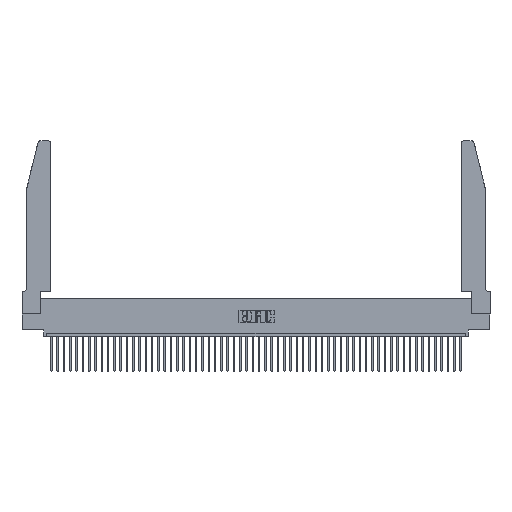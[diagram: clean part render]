
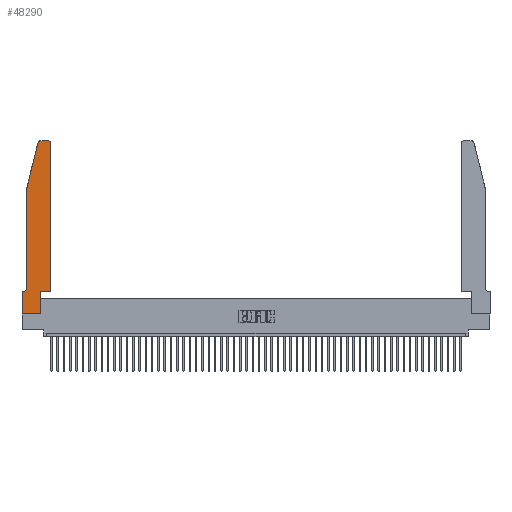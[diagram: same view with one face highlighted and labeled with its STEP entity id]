
A CAD part, top view. The second image highlights one B-rep face of the part: STEP entity #48290.
In plain terms, the highlighted planar face has unit normal (0, 0, 1).
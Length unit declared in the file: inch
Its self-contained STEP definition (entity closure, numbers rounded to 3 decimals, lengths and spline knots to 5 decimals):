
#270 = VECTOR ( 'NONE', #30707, 39.37008 ) ;
#1154 = DIRECTION ( 'NONE',  ( -1., 0., 0. ) ) ;
#1401 = LINE ( 'NONE', #25090, #33498 ) ;
#1733 = CARTESIAN_POINT ( 'NONE',  ( 0.2865, 0.35, 0.37 ) ) ;
#1856 = VERTEX_POINT ( 'NONE', #25695 ) ;
#2236 = DIRECTION ( 'NONE',  ( 1., 0., 0. ) ) ;
#2900 = CARTESIAN_POINT ( 'NONE',  ( 0.0755, 2., 0.37 ) ) ;
#3013 = ORIENTED_EDGE ( 'NONE', *, *, #14143, .T. ) ;
#3440 = DIRECTION ( 'NONE',  ( 0., -1., 0. ) ) ;
#4960 = AXIS2_PLACEMENT_3D ( 'NONE', #7551, #12143, #24899 ) ;
#5431 = EDGE_CURVE ( 'NONE', #17970, #30883, #45743, .T. ) ;
#6636 = DIRECTION ( 'NONE',  ( 0., 0., 1. ) ) ;
#7530 = VERTEX_POINT ( 'NONE', #18806 ) ;
#7551 = CARTESIAN_POINT ( 'NONE',  ( 0.284, 2.72, 0.37 ) ) ;
#8473 = CARTESIAN_POINT ( 'NONE',  ( 0.2605, 2.75, 0.37 ) ) ;
#9824 = ORIENTED_EDGE ( 'NONE', *, *, #10582, .T. ) ;
#10582 = EDGE_CURVE ( 'NONE', #50587, #1856, #40303, .T. ) ;
#10866 = ORIENTED_EDGE ( 'NONE', *, *, #5431, .T. ) ;
#11333 = CARTESIAN_POINT ( 'NONE',  ( 0.0055, 0.42, 0.37 ) ) ;
#12091 = CARTESIAN_POINT ( 'NONE',  ( 0.2865, 0.35, 0.37 ) ) ;
#12143 = DIRECTION ( 'NONE',  ( 0., 0., 1. ) ) ;
#13010 = CARTESIAN_POINT ( 'NONE',  ( 0., 0.35, 0.37 ) ) ;
#13151 = EDGE_CURVE ( 'NONE', #7530, #50587, #1401, .T. ) ;
#13411 = VECTOR ( 'NONE', #21509, 39.37008 ) ;
#13503 = CARTESIAN_POINT ( 'NONE',  ( 0.25487, 2.72718, 0.37 ) ) ;
#13522 = DIRECTION ( 'NONE',  ( 1., 0., 0. ) ) ;
#14143 = EDGE_CURVE ( 'NONE', #32393, #18899, #32865, .T. ) ;
#14717 = DIRECTION ( 'NONE',  ( 0., 0., -1. ) ) ;
#15496 = ORIENTED_EDGE ( 'NONE', *, *, #30659, .T. ) ;
#16083 = CARTESIAN_POINT ( 'NONE',  ( 0.4505, 2.72, 0.37 ) ) ;
#16357 = CARTESIAN_POINT ( 'NONE',  ( 0.0755, 0.42, 0.37 ) ) ;
#16364 = EDGE_CURVE ( 'NONE', #30883, #48592, #29950, .T. ) ;
#16463 = EDGE_CURVE ( 'NONE', #18875, #7530, #46113, .T. ) ;
#16797 = CARTESIAN_POINT ( 'NONE',  ( 0.4205, 2.75, 0.37 ) ) ;
#17970 = VERTEX_POINT ( 'NONE', #22312 ) ;
#18290 = LINE ( 'NONE', #36904, #47576 ) ;
#18806 = CARTESIAN_POINT ( 'NONE',  ( 0.0055, 0.35, 0.37 ) ) ;
#18875 = VERTEX_POINT ( 'NONE', #16357 ) ;
#18899 = VERTEX_POINT ( 'NONE', #48061 ) ;
#19229 = VERTEX_POINT ( 'NONE', #16797 ) ;
#19239 = ORIENTED_EDGE ( 'NONE', *, *, #16463, .T. ) ;
#19717 = CARTESIAN_POINT ( 'NONE',  ( 0.4505, 0.35, 0.37 ) ) ;
#19739 = EDGE_CURVE ( 'NONE', #48592, #18875, #33298, .T. ) ;
#20328 = LINE ( 'NONE', #8473, #27850 ) ;
#20359 = DIRECTION ( 'NONE',  ( 0., -1., 0. ) ) ;
#20773 = EDGE_CURVE ( 'NONE', #1856, #48542, #18290, .T. ) ;
#20975 = CARTESIAN_POINT ( 'NONE',  ( 0., 0.35, 0.37 ) ) ;
#21509 = DIRECTION ( 'NONE',  ( 0., 1., 0. ) ) ;
#21922 = DIRECTION ( 'NONE',  ( 1., 0., 0. ) ) ;
#22312 = CARTESIAN_POINT ( 'NONE',  ( 0.284, 2.75, 0.37 ) ) ;
#22869 = CARTESIAN_POINT ( 'NONE',  ( 0.2865, 0., 0.37 ) ) ;
#23651 = DIRECTION ( 'NONE',  ( -1., 0., 0. ) ) ;
#24859 = ORIENTED_EDGE ( 'NONE', *, *, #16364, .T. ) ;
#24899 = DIRECTION ( 'NONE',  ( 1., 0., 0. ) ) ;
#25090 = CARTESIAN_POINT ( 'NONE',  ( 0.0755, 0.35, 0.37 ) ) ;
#25695 = CARTESIAN_POINT ( 'NONE',  ( 0., 0., 0.37 ) ) ;
#26265 = ORIENTED_EDGE ( 'NONE', *, *, #19739, .T. ) ;
#26430 = AXIS2_PLACEMENT_3D ( 'NONE', #13010, #44469, #33238 ) ;
#27118 = LINE ( 'NONE', #1733, #13411 ) ;
#27508 = VECTOR ( 'NONE', #47598, 39.37008 ) ;
#27850 = VECTOR ( 'NONE', #23651, 39.37008 ) ;
#29950 = LINE ( 'NONE', #2900, #270 ) ;
#30659 = EDGE_CURVE ( 'NONE', #18899, #50947, #45557, .T. ) ;
#30707 = DIRECTION ( 'NONE',  ( -0.239, -0.971, 0. ) ) ;
#30883 = VERTEX_POINT ( 'NONE', #13503 ) ;
#31406 = CARTESIAN_POINT ( 'NONE',  ( 0., 0., 0.37 ) ) ;
#32059 = EDGE_CURVE ( 'NONE', #50947, #19229, #46003, .T. ) ;
#32393 = VERTEX_POINT ( 'NONE', #12091 ) ;
#32865 = LINE ( 'NONE', #33632, #38510 ) ;
#33238 = DIRECTION ( 'NONE',  ( 1., 0., 0. ) ) ;
#33298 = LINE ( 'NONE', #43809, #48322 ) ;
#33498 = VECTOR ( 'NONE', #1154, 39.37008 ) ;
#33632 = CARTESIAN_POINT ( 'NONE',  ( 0.4505, 0.35, 0.37 ) ) ;
#33958 = ORIENTED_EDGE ( 'NONE', *, *, #47804, .T. ) ;
#35311 = ORIENTED_EDGE ( 'NONE', *, *, #32059, .T. ) ;
#36904 = CARTESIAN_POINT ( 'NONE',  ( 0., 0., 0.37 ) ) ;
#37215 = ORIENTED_EDGE ( 'NONE', *, *, #13151, .T. ) ;
#38506 = CARTESIAN_POINT ( 'NONE',  ( 0.0755, 2., 0.37 ) ) ;
#38510 = VECTOR ( 'NONE', #2236, 39.37008 ) ;
#38785 = ORIENTED_EDGE ( 'NONE', *, *, #20773, .T. ) ;
#39945 = ORIENTED_EDGE ( 'NONE', *, *, #46332, .T. ) ;
#40303 = LINE ( 'NONE', #31406, #47049 ) ;
#43061 = DIRECTION ( 'NONE',  ( -1., 0., 0. ) ) ;
#43184 = FACE_OUTER_BOUND ( 'NONE', #43861, .T. ) ;
#43809 = CARTESIAN_POINT ( 'NONE',  ( 0.0755, 2., 0.37 ) ) ;
#43861 = EDGE_LOOP ( 'NONE', ( #39945, #10866, #24859, #26265, #19239, #37215, #9824, #38785, #33958, #3013, #15496, #35311 ) ) ;
#44150 = AXIS2_PLACEMENT_3D ( 'NONE', #11333, #14717, #43061 ) ;
#44469 = DIRECTION ( 'NONE',  ( 0., 0., 1. ) ) ;
#44638 = AXIS2_PLACEMENT_3D ( 'NONE', #50156, #6636, #21922 ) ;
#45557 = LINE ( 'NONE', #19717, #27508 ) ;
#45743 = CIRCLE ( 'NONE', #4960, 0.03 ) ;
#46003 = CIRCLE ( 'NONE', #44638, 0.03 ) ;
#46113 = CIRCLE ( 'NONE', #44150, 0.07 ) ;
#46332 = EDGE_CURVE ( 'NONE', #19229, #17970, #20328, .T. ) ;
#47049 = VECTOR ( 'NONE', #3440, 39.37008 ) ;
#47576 = VECTOR ( 'NONE', #13522, 39.37008 ) ;
#47598 = DIRECTION ( 'NONE',  ( 0., 1., 0. ) ) ;
#47804 = EDGE_CURVE ( 'NONE', #48542, #32393, #27118, .T. ) ;
#48061 = CARTESIAN_POINT ( 'NONE',  ( 0.4505, 0.35, 0.37 ) ) ;
#48290 = ADVANCED_FACE ( 'NONE', ( #43184 ), #48634, .T. ) ;
#48322 = VECTOR ( 'NONE', #20359, 39.37008 ) ;
#48542 = VERTEX_POINT ( 'NONE', #22869 ) ;
#48592 = VERTEX_POINT ( 'NONE', #38506 ) ;
#48634 = PLANE ( 'NONE',  #26430 ) ;
#50156 = CARTESIAN_POINT ( 'NONE',  ( 0.4205, 2.72, 0.37 ) ) ;
#50587 = VERTEX_POINT ( 'NONE', #20975 ) ;
#50947 = VERTEX_POINT ( 'NONE', #16083 ) ;
